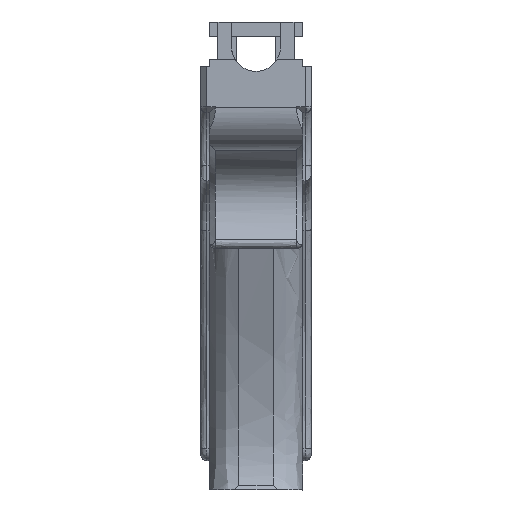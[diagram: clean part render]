
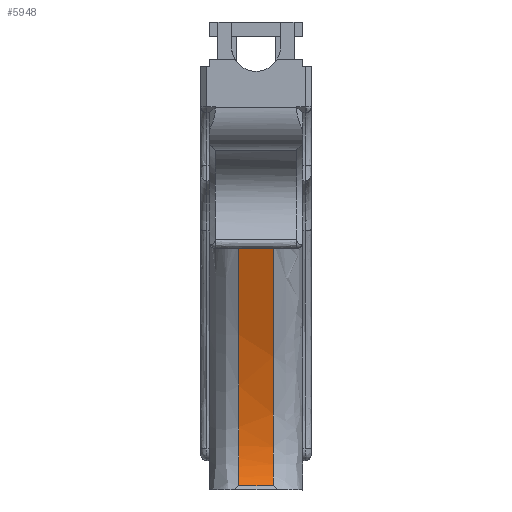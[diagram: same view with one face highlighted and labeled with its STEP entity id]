
A CAD part, front view. The second image highlights one B-rep face of the part: STEP entity #5948.
In plain terms, the highlighted free-form (B-spline) face has degree [5, 1] with [15, 2] control points.
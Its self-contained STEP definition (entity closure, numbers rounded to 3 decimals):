
#29=(
BOUNDED_SURFACE()
B_SPLINE_SURFACE(5,1,((#11396,#11397),(#11398,#11399),(#11400,#11401),(#11402,
#11403),(#11404,#11405),(#11406,#11407),(#11408,#11409),(#11410,#11411),
(#11412,#11413),(#11414,#11415),(#11416,#11417),(#11418,#11419),(#11420,
#11421),(#11422,#11423),(#11424,#11425)),.UNSPECIFIED.,.F.,.F.,.F.)
B_SPLINE_SURFACE_WITH_KNOTS((6,1,1,1,1,1,1,1,1,1,6),(2,2),(0.,0.1,0.2,0.3,
0.4,0.5,0.6,0.7,0.8,0.9,1.),(0.,4.5),.UNSPECIFIED.)
GEOMETRIC_REPRESENTATION_ITEM()
RATIONAL_B_SPLINE_SURFACE(((1.,1.),(1.,1.),(1.,1.),(1.,1.),(1.,1.),(1.,
1.),(1.,1.),(1.,1.),(1.,1.),(1.,1.),(1.,1.),(1.,1.),(1.,1.),(1.,1.),(1.,
1.)))
REPRESENTATION_ITEM('')
SURFACE()
);
#679=FACE_OUTER_BOUND('',#1021,.T.);
#1021=EDGE_LOOP('',(#5076,#5077,#5078,#5079));
#2398=B_SPLINE_CURVE_WITH_KNOTS('',3,(#11291,#11292,#11293,#11294),
 .UNSPECIFIED.,.F.,.F.,(4,4),(-1.09,-0.5),.UNSPECIFIED.);
#2399=B_SPLINE_CURVE_WITH_KNOTS('',3,(#11370,#11371,#11372,#11373,#11374,
#11375,#11376,#11377,#11378,#11379),.UNSPECIFIED.,.F.,.F.,(4,1,1,1,1,1,
1,4),(0.076,1.482,2.186,2.537,
2.889,3.593,4.296,4.886),
 .UNSPECIFIED.);
#2401=B_SPLINE_CURVE_WITH_KNOTS('',3,(#11427,#11428,#11429,#11430,#11431,
#11432,#11433,#11434,#11435,#11436,#11437,#11438),.UNSPECIFIED.,.F.,.F.,
(4,1,1,1,1,1,1,1,1,4),(0.113,0.703,1.055,
1.407,2.11,2.814,3.165,3.517,
4.221,4.924),.UNSPECIFIED.);
#2402=B_SPLINE_CURVE_WITH_KNOTS('',3,(#11439,#11440,#11441,#11442),
 .UNSPECIFIED.,.F.,.F.,(4,4),(-1.09,-0.5),.UNSPECIFIED.);
#2926=VERTEX_POINT('',#11270);
#2927=VERTEX_POINT('',#11289);
#2928=VERTEX_POINT('',#11369);
#2929=VERTEX_POINT('',#11426);
#3707=EDGE_CURVE('',#2927,#2926,#2398,.T.);
#3709=EDGE_CURVE('',#2926,#2928,#2399,.T.);
#3711=EDGE_CURVE('',#2929,#2927,#2401,.T.);
#3712=EDGE_CURVE('',#2928,#2929,#2402,.T.);
#5076=ORIENTED_EDGE('',*,*,#3707,.F.);
#5077=ORIENTED_EDGE('',*,*,#3711,.F.);
#5078=ORIENTED_EDGE('',*,*,#3712,.F.);
#5079=ORIENTED_EDGE('',*,*,#3709,.F.);
#5948=ADVANCED_FACE('',(#679),#29,.F.);
#11270=CARTESIAN_POINT('',(10.9,-37.342,-27.594));
#11289=CARTESIAN_POINT('',(5.,-37.342,-27.594));
#11291=CARTESIAN_POINT('Ctrl Pts',(5.,-37.342,-27.594));
#11292=CARTESIAN_POINT('Ctrl Pts',(6.967,-37.342,-27.594));
#11293=CARTESIAN_POINT('Ctrl Pts',(8.933,-37.342,-27.594));
#11294=CARTESIAN_POINT('Ctrl Pts',(10.9,-37.342,-27.594));
#11369=CARTESIAN_POINT('',(10.9,-29.623,-69.406));
#11370=CARTESIAN_POINT('Ctrl Pts',(10.9,-37.342,-27.594));
#11371=CARTESIAN_POINT('Ctrl Pts',(10.9,-35.653,-31.896));
#11372=CARTESIAN_POINT('Ctrl Pts',(10.9,-33.249,-38.38));
#11373=CARTESIAN_POINT('Ctrl Pts',(10.9,-30.86,-45.979));
#11374=CARTESIAN_POINT('Ctrl Pts',(10.9,-29.683,-50.314));
#11375=CARTESIAN_POINT('Ctrl Pts',(10.9,-28.677,-54.62));
#11376=CARTESIAN_POINT('Ctrl Pts',(10.9,-27.819,-59.909));
#11377=CARTESIAN_POINT('Ctrl Pts',(10.9,-27.943,-65.457));
#11378=CARTESIAN_POINT('Ctrl Pts',(10.9,-28.97,-68.314));
#11379=CARTESIAN_POINT('Ctrl Pts',(10.9,-29.624,-69.405));
#11396=CARTESIAN_POINT('Ctrl Pts',(0.,-30.016,
-70.003));
#11397=CARTESIAN_POINT('Ctrl Pts',(45.,-30.016,-70.003));
#11398=CARTESIAN_POINT('Ctrl Pts',(0.,-29.748,
-69.63));
#11399=CARTESIAN_POINT('Ctrl Pts',(45.,-29.748,-69.63));
#11400=CARTESIAN_POINT('Ctrl Pts',(0.,-29.253,
-68.836));
#11401=CARTESIAN_POINT('Ctrl Pts',(45.,-29.253,-68.836));
#11402=CARTESIAN_POINT('Ctrl Pts',(0.,-28.637,
-67.498));
#11403=CARTESIAN_POINT('Ctrl Pts',(45.,-28.637,-67.498));
#11404=CARTESIAN_POINT('Ctrl Pts',(0.,-28.071,
-65.416));
#11405=CARTESIAN_POINT('Ctrl Pts',(45.,-28.071,-65.416));
#11406=CARTESIAN_POINT('Ctrl Pts',(0.,-27.812,
-62.291));
#11407=CARTESIAN_POINT('Ctrl Pts',(45.,-27.812,-62.291));
#11408=CARTESIAN_POINT('Ctrl Pts',(0.,-28.022,
-58.621));
#11409=CARTESIAN_POINT('Ctrl Pts',(45.,-28.022,-58.621));
#11410=CARTESIAN_POINT('Ctrl Pts',(0.,-28.695,
-54.412));
#11411=CARTESIAN_POINT('Ctrl Pts',(45.,-28.695,-54.412));
#11412=CARTESIAN_POINT('Ctrl Pts',(0.,-29.793,
-49.709));
#11413=CARTESIAN_POINT('Ctrl Pts',(45.,-29.793,-49.709));
#11414=CARTESIAN_POINT('Ctrl Pts',(0.,-31.267,
-44.567));
#11415=CARTESIAN_POINT('Ctrl Pts',(45.,-31.267,-44.567));
#11416=CARTESIAN_POINT('Ctrl Pts',(0.,-33.073,
-39.04));
#11417=CARTESIAN_POINT('Ctrl Pts',(45.,-33.073,-39.04));
#11418=CARTESIAN_POINT('Ctrl Pts',(0.,-34.754,
-34.343));
#11419=CARTESIAN_POINT('Ctrl Pts',(45.,-34.754,-34.343));
#11420=CARTESIAN_POINT('Ctrl Pts',(0.,-36.138,
-30.676));
#11421=CARTESIAN_POINT('Ctrl Pts',(45.,-36.138,-30.676));
#11422=CARTESIAN_POINT('Ctrl Pts',(0.,-37.114,
-28.169));
#11423=CARTESIAN_POINT('Ctrl Pts',(45.,-37.114,-28.169));
#11424=CARTESIAN_POINT('Ctrl Pts',(0.,-37.616,
-26.9));
#11425=CARTESIAN_POINT('Ctrl Pts',(45.,-37.616,-26.9));
#11426=CARTESIAN_POINT('',(5.,-29.623,-69.406));
#11427=CARTESIAN_POINT('Ctrl Pts',(5.,-29.624,-69.405));
#11428=CARTESIAN_POINT('Ctrl Pts',(5.,-28.97,-68.314));
#11429=CARTESIAN_POINT('Ctrl Pts',(5.,-28.224,-66.235));
#11430=CARTESIAN_POINT('Ctrl Pts',(5.,-27.883,-62.836));
#11431=CARTESIAN_POINT('Ctrl Pts',(5.,-27.992,-58.854));
#11432=CARTESIAN_POINT('Ctrl Pts',(5.,-28.848,-53.559));
#11433=CARTESIAN_POINT('Ctrl Pts',(5.,-30.241,-48.143));
#11434=CARTESIAN_POINT('Ctrl Pts',(5.,-31.544,-43.804));
#11435=CARTESIAN_POINT('Ctrl Pts',(5.,-32.948,-39.467));
#11436=CARTESIAN_POINT('Ctrl Pts',(5.,-34.854,-34.059));
#11437=CARTESIAN_POINT('Ctrl Pts',(5.,-36.497,-29.745));
#11438=CARTESIAN_POINT('Ctrl Pts',(5.,-37.342,-27.594));
#11439=CARTESIAN_POINT('Ctrl Pts',(10.9,-29.623,-69.406));
#11440=CARTESIAN_POINT('Ctrl Pts',(8.933,-29.623,-69.406));
#11441=CARTESIAN_POINT('Ctrl Pts',(6.967,-29.623,-69.406));
#11442=CARTESIAN_POINT('Ctrl Pts',(5.,-29.623,-69.406));
